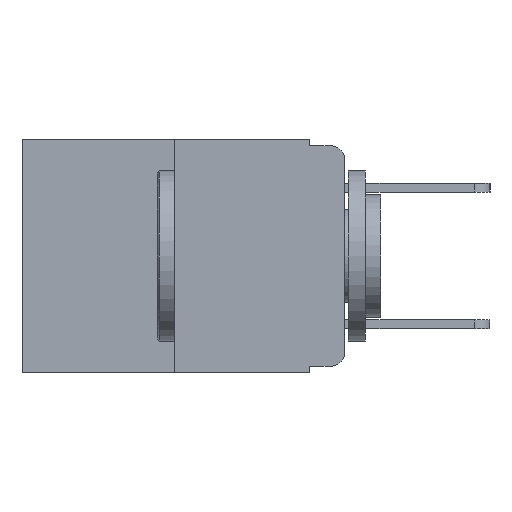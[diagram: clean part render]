
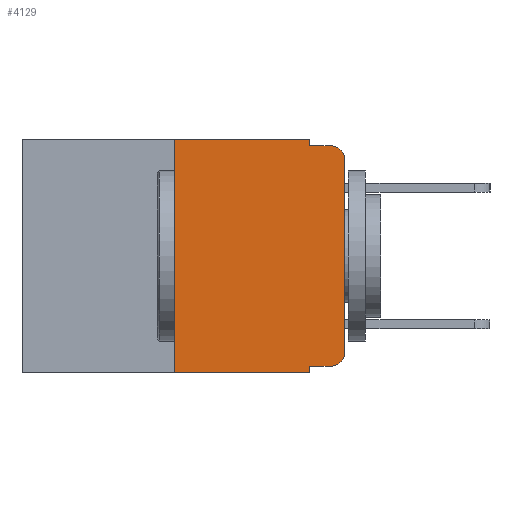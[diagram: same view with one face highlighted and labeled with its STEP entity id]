
A CAD part, left-side view. The second image highlights one B-rep face of the part: STEP entity #4129.
In plain terms, the highlighted planar face has unit normal (-1, 0, 0).
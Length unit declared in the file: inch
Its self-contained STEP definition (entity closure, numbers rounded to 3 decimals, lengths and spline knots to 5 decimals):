
#306 = VERTEX_POINT ( 'NONE', #10399 ) ;
#575 = LINE ( 'NONE', #11367, #9949 ) ;
#676 = CARTESIAN_POINT ( 'NONE',  ( 0., 0.25, -0.343 ) ) ;
#718 = DIRECTION ( 'NONE',  ( 0., 0., -1. ) ) ;
#856 = VERTEX_POINT ( 'NONE', #9073 ) ;
#1033 = CARTESIAN_POINT ( 'NONE',  ( 0., 0.051, 0. ) ) ;
#1045 = VERTEX_POINT ( 'NONE', #10701 ) ;
#1290 = CIRCLE ( 'NONE', #10157, 0.02 ) ;
#1483 = VERTEX_POINT ( 'NONE', #7881 ) ;
#1539 = LINE ( 'NONE', #3795, #4497 ) ;
#1644 = CARTESIAN_POINT ( 'NONE',  ( 0., 0.473, 0. ) ) ;
#1753 = VECTOR ( 'NONE', #13430, 39.37008 ) ;
#2105 = DIRECTION ( 'NONE',  ( 0., 0., -1. ) ) ;
#2156 = ORIENTED_EDGE ( 'NONE', *, *, #9231, .F. ) ;
#2314 = CARTESIAN_POINT ( 'NONE',  ( 0., 0.051, -0.333 ) ) ;
#2948 = DIRECTION ( 'NONE',  ( 1., 0., 0. ) ) ;
#3261 = CARTESIAN_POINT ( 'NONE',  ( 0., 0.051, -0.333 ) ) ;
#3630 = EDGE_CURVE ( 'NONE', #1483, #5621, #10947, .T. ) ;
#3795 = CARTESIAN_POINT ( 'NONE',  ( 0., 0.051, -0.01 ) ) ;
#3929 = VECTOR ( 'NONE', #2105, 39.37008 ) ;
#4083 = VERTEX_POINT ( 'NONE', #12035 ) ;
#4129 = ADVANCED_FACE ( 'NONE', ( #8305 ), #12079, .F. ) ;
#4497 = VECTOR ( 'NONE', #9718, 39.37008 ) ;
#4502 = DIRECTION ( 'NONE',  ( 0., 0., 1. ) ) ;
#4536 = VECTOR ( 'NONE', #6196, 39.37008 ) ;
#4676 = EDGE_LOOP ( 'NONE', ( #12804, #10814, #2156, #12099, #8009, #4736, #7065, #13844, #7238, #14304 ) ) ;
#4736 = ORIENTED_EDGE ( 'NONE', *, *, #6909, .F. ) ;
#4788 = AXIS2_PLACEMENT_3D ( 'NONE', #14516, #8139, #718 ) ;
#4921 = LINE ( 'NONE', #4999, #4536 ) ;
#4999 = CARTESIAN_POINT ( 'NONE',  ( 0., 0.473, -0.343 ) ) ;
#5305 = EDGE_CURVE ( 'NONE', #7672, #1483, #12818, .T. ) ;
#5395 = VECTOR ( 'NONE', #9416, 39.37008 ) ;
#5621 = VERTEX_POINT ( 'NONE', #13333 ) ;
#6097 = EDGE_CURVE ( 'NONE', #7672, #306, #8793, .T. ) ;
#6123 = EDGE_CURVE ( 'NONE', #6935, #306, #4921, .T. ) ;
#6196 = DIRECTION ( 'NONE',  ( 0., -1., 0. ) ) ;
#6282 = DIRECTION ( 'NONE',  ( -1., 0., 0. ) ) ;
#6909 = EDGE_CURVE ( 'NONE', #6935, #856, #13583, .T. ) ;
#6935 = VERTEX_POINT ( 'NONE', #676 ) ;
#7065 = ORIENTED_EDGE ( 'NONE', *, *, #6123, .T. ) ;
#7169 = LINE ( 'NONE', #12440, #3929 ) ;
#7238 = ORIENTED_EDGE ( 'NONE', *, *, #5305, .T. ) ;
#7374 = VECTOR ( 'NONE', #14650, 39.37008 ) ;
#7672 = VERTEX_POINT ( 'NONE', #3261 ) ;
#7881 = CARTESIAN_POINT ( 'NONE',  ( 0., 0.02, -0.333 ) ) ;
#8009 = ORIENTED_EDGE ( 'NONE', *, *, #10827, .F. ) ;
#8139 = DIRECTION ( 'NONE',  ( -1., 0., 0. ) ) ;
#8185 = VERTEX_POINT ( 'NONE', #10070 ) ;
#8227 = CARTESIAN_POINT ( 'NONE',  ( 0., 0.473, 0. ) ) ;
#8305 = FACE_OUTER_BOUND ( 'NONE', #4676, .T. ) ;
#8452 = EDGE_CURVE ( 'NONE', #4083, #13349, #7169, .T. ) ;
#8793 = LINE ( 'NONE', #1033, #14107 ) ;
#9073 = CARTESIAN_POINT ( 'NONE',  ( 0., 0.25, 0. ) ) ;
#9231 = EDGE_CURVE ( 'NONE', #13349, #8185, #1539, .T. ) ;
#9416 = DIRECTION ( 'NONE',  ( 0., -1., 0. ) ) ;
#9566 = DIRECTION ( 'NONE',  ( 0., 0., -1. ) ) ;
#9718 = DIRECTION ( 'NONE',  ( 0., -1., 0. ) ) ;
#9949 = VECTOR ( 'NONE', #4502, 39.37008 ) ;
#9974 = EDGE_CURVE ( 'NONE', #1045, #8185, #1290, .T. ) ;
#10070 = CARTESIAN_POINT ( 'NONE',  ( 0., 0.02, -0.01 ) ) ;
#10157 = AXIS2_PLACEMENT_3D ( 'NONE', #12896, #6282, #13937 ) ;
#10399 = CARTESIAN_POINT ( 'NONE',  ( 0., 0.051, -0.343 ) ) ;
#10701 = CARTESIAN_POINT ( 'NONE',  ( 0., 0., -0.03 ) ) ;
#10706 = EDGE_CURVE ( 'NONE', #5621, #1045, #575, .T. ) ;
#10711 = AXIS2_PLACEMENT_3D ( 'NONE', #1644, #2948, #11091 ) ;
#10814 = ORIENTED_EDGE ( 'NONE', *, *, #9974, .T. ) ;
#10827 = EDGE_CURVE ( 'NONE', #856, #4083, #14182, .T. ) ;
#10947 = CIRCLE ( 'NONE', #4788, 0.02 ) ;
#11091 = DIRECTION ( 'NONE',  ( 0., 0., -1. ) ) ;
#11352 = CARTESIAN_POINT ( 'NONE',  ( 0., 0.25, 0. ) ) ;
#11367 = CARTESIAN_POINT ( 'NONE',  ( 0., 0., 0. ) ) ;
#11751 = CARTESIAN_POINT ( 'NONE',  ( 0., 0.051, -0.01 ) ) ;
#12035 = CARTESIAN_POINT ( 'NONE',  ( 0., 0.051, 0. ) ) ;
#12079 = PLANE ( 'NONE',  #10711 ) ;
#12099 = ORIENTED_EDGE ( 'NONE', *, *, #8452, .F. ) ;
#12440 = CARTESIAN_POINT ( 'NONE',  ( 0., 0.051, 0. ) ) ;
#12804 = ORIENTED_EDGE ( 'NONE', *, *, #10706, .T. ) ;
#12818 = LINE ( 'NONE', #2314, #7374 ) ;
#12896 = CARTESIAN_POINT ( 'NONE',  ( 0., 0.02, -0.03 ) ) ;
#13333 = CARTESIAN_POINT ( 'NONE',  ( 0., 0., -0.313 ) ) ;
#13349 = VERTEX_POINT ( 'NONE', #11751 ) ;
#13430 = DIRECTION ( 'NONE',  ( 0., 0., 1. ) ) ;
#13583 = LINE ( 'NONE', #11352, #1753 ) ;
#13844 = ORIENTED_EDGE ( 'NONE', *, *, #6097, .F. ) ;
#13937 = DIRECTION ( 'NONE',  ( 0., 0., -1. ) ) ;
#14107 = VECTOR ( 'NONE', #9566, 39.37008 ) ;
#14182 = LINE ( 'NONE', #8227, #5395 ) ;
#14304 = ORIENTED_EDGE ( 'NONE', *, *, #3630, .T. ) ;
#14516 = CARTESIAN_POINT ( 'NONE',  ( 0., 0.02, -0.313 ) ) ;
#14650 = DIRECTION ( 'NONE',  ( 0., -1., 0. ) ) ;
